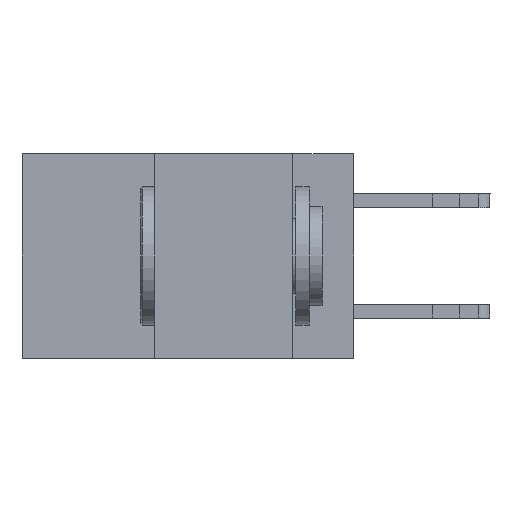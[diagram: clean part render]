
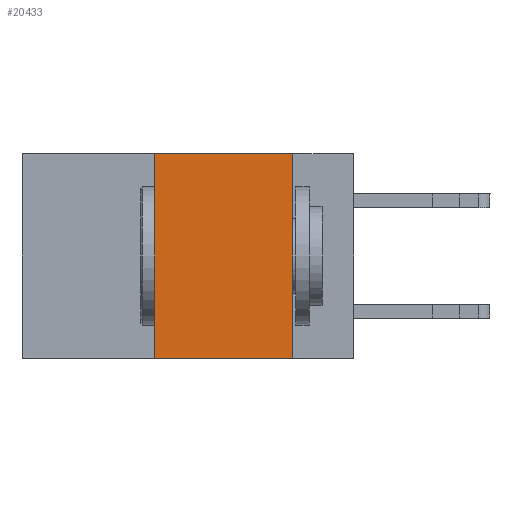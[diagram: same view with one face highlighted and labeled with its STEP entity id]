
A CAD part, left-side view. The second image highlights one B-rep face of the part: STEP entity #20433.
In plain terms, the highlighted planar face has unit normal (-1, 0, 0).
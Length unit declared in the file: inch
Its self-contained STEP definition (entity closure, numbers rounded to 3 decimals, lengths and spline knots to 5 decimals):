
#345 = PLANE ( 'NONE',  #21663 ) ;
#711 = EDGE_CURVE ( 'NONE', #2079, #10682, #12002, .T. ) ;
#1603 = EDGE_CURVE ( 'NONE', #10468, #19107, #9586, .T. ) ;
#1916 = ORIENTED_EDGE ( 'NONE', *, *, #18395, .F. ) ;
#1936 = LINE ( 'NONE', #3419, #11016 ) ;
#2051 = DIRECTION ( 'NONE',  ( 0., -1., 0. ) ) ;
#2079 = VERTEX_POINT ( 'NONE', #14420 ) ;
#3419 = CARTESIAN_POINT ( 'NONE',  ( 0., 0.36, 0. ) ) ;
#4666 = DIRECTION ( 'NONE',  ( 0., -1., 0. ) ) ;
#5052 = VECTOR ( 'NONE', #2051, 39.37008 ) ;
#6467 = VECTOR ( 'NONE', #4666, 39.37008 ) ;
#6687 = CARTESIAN_POINT ( 'NONE',  ( 0., 0.11, 0. ) ) ;
#6939 = CARTESIAN_POINT ( 'NONE',  ( 0., 0.11, -0.37 ) ) ;
#8704 = EDGE_LOOP ( 'NONE', ( #9990, #16032, #1916, #8735 ) ) ;
#8735 = ORIENTED_EDGE ( 'NONE', *, *, #711, .T. ) ;
#9586 = LINE ( 'NONE', #20672, #5052 ) ;
#9990 = ORIENTED_EDGE ( 'NONE', *, *, #14469, .F. ) ;
#10468 = VERTEX_POINT ( 'NONE', #14695 ) ;
#10682 = VERTEX_POINT ( 'NONE', #6939 ) ;
#11016 = VECTOR ( 'NONE', #21822, 39.37008 ) ;
#11571 = CARTESIAN_POINT ( 'NONE',  ( 0., 0.6, -0.37 ) ) ;
#12002 = LINE ( 'NONE', #11571, #6467 ) ;
#12096 = DIRECTION ( 'NONE',  ( 1., 0., 0. ) ) ;
#12739 = VECTOR ( 'NONE', #16208, 39.37008 ) ;
#13805 = DIRECTION ( 'NONE',  ( 0., 0., -1. ) ) ;
#14420 = CARTESIAN_POINT ( 'NONE',  ( 0., 0.36, -0.37 ) ) ;
#14469 = EDGE_CURVE ( 'NONE', #19107, #10682, #19377, .T. ) ;
#14695 = CARTESIAN_POINT ( 'NONE',  ( 0., 0.36, 0. ) ) ;
#16032 = ORIENTED_EDGE ( 'NONE', *, *, #1603, .F. ) ;
#16208 = DIRECTION ( 'NONE',  ( 0., 0., -1. ) ) ;
#17532 = FACE_OUTER_BOUND ( 'NONE', #8704, .T. ) ;
#18395 = EDGE_CURVE ( 'NONE', #2079, #10468, #1936, .T. ) ;
#18845 = CARTESIAN_POINT ( 'NONE',  ( 0., 0.6, 0. ) ) ;
#19107 = VERTEX_POINT ( 'NONE', #6687 ) ;
#19377 = LINE ( 'NONE', #21243, #12739 ) ;
#20433 = ADVANCED_FACE ( 'NONE', ( #17532 ), #345, .F. ) ;
#20672 = CARTESIAN_POINT ( 'NONE',  ( 0., 0.6, 0. ) ) ;
#21243 = CARTESIAN_POINT ( 'NONE',  ( 0., 0.11, 0. ) ) ;
#21663 = AXIS2_PLACEMENT_3D ( 'NONE', #18845, #12096, #13805 ) ;
#21822 = DIRECTION ( 'NONE',  ( 0., 0., 1. ) ) ;
